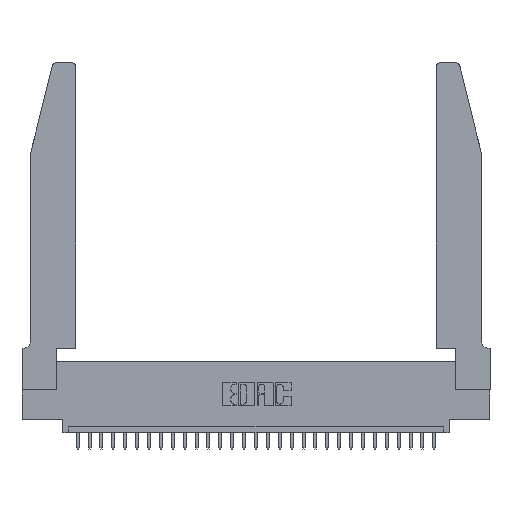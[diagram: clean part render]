
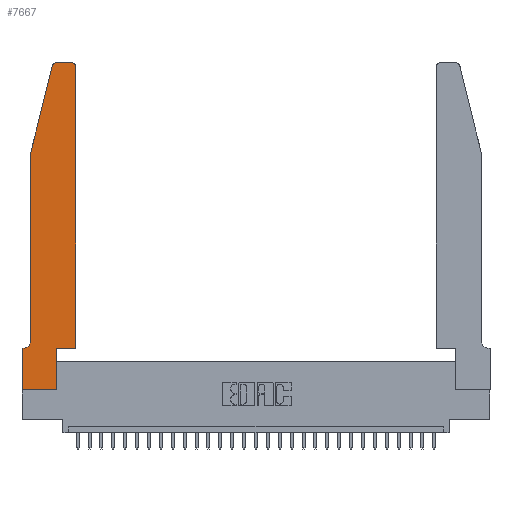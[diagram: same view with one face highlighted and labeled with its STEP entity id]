
A CAD part, top view. The second image highlights one B-rep face of the part: STEP entity #7667.
In plain terms, the highlighted planar face has unit normal (0, 0, 1).
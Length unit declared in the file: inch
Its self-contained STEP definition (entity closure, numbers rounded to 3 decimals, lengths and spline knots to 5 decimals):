
#286 = CARTESIAN_POINT ( 'NONE',  ( 0.2865, 0.35, 0.37 ) ) ;
#939 = VERTEX_POINT ( 'NONE', #19183 ) ;
#998 = ORIENTED_EDGE ( 'NONE', *, *, #2613, .T. ) ;
#1037 = DIRECTION ( 'NONE',  ( 0., -1., 0. ) ) ;
#2097 = DIRECTION ( 'NONE',  ( -1., 0., 0. ) ) ;
#2225 = DIRECTION ( 'NONE',  ( -1., 0., 0. ) ) ;
#2613 = EDGE_CURVE ( 'NONE', #14216, #12177, #20416, .T. ) ;
#2931 = CARTESIAN_POINT ( 'NONE',  ( 0.4205, 2.72, 0.37 ) ) ;
#3018 = CIRCLE ( 'NONE', #9901, 0.03 ) ;
#3137 = DIRECTION ( 'NONE',  ( 0., 1., 0. ) ) ;
#3200 = VECTOR ( 'NONE', #1037, 39.37008 ) ;
#3619 = DIRECTION ( 'NONE',  ( 0., 0., -1. ) ) ;
#3767 = DIRECTION ( 'NONE',  ( 1., 0., 0. ) ) ;
#3789 = EDGE_LOOP ( 'NONE', ( #17367, #20407, #10611, #998, #13333, #12583, #29360, #24971, #9728, #26779, #10005, #27233 ) ) ;
#3909 = CARTESIAN_POINT ( 'NONE',  ( 0.2865, 0., 0.37 ) ) ;
#3912 = CARTESIAN_POINT ( 'NONE',  ( 0.0755, 2., 0.37 ) ) ;
#4201 = CARTESIAN_POINT ( 'NONE',  ( 0., 0., 0.37 ) ) ;
#4343 = CARTESIAN_POINT ( 'NONE',  ( 0.4505, 0.35, 0.37 ) ) ;
#4499 = LINE ( 'NONE', #4343, #17440 ) ;
#5160 = VECTOR ( 'NONE', #19222, 39.37008 ) ;
#5215 = DIRECTION ( 'NONE',  ( 1., 0., 0. ) ) ;
#5331 = EDGE_CURVE ( 'NONE', #27801, #14195, #3018, .T. ) ;
#5688 = LINE ( 'NONE', #21274, #18525 ) ;
#6312 = CARTESIAN_POINT ( 'NONE',  ( 0.4505, 0.35, 0.37 ) ) ;
#6577 = VERTEX_POINT ( 'NONE', #15062 ) ;
#7338 = CARTESIAN_POINT ( 'NONE',  ( 0.284, 2.75, 0.37 ) ) ;
#7594 = DIRECTION ( 'NONE',  ( 1., 0., 0. ) ) ;
#7667 = ADVANCED_FACE ( 'NONE', ( #29215 ), #26389, .T. ) ;
#8290 = EDGE_CURVE ( 'NONE', #15858, #14216, #28092, .T. ) ;
#8324 = EDGE_CURVE ( 'NONE', #6577, #10058, #9838, .T. ) ;
#8410 = DIRECTION ( 'NONE',  ( 0., 0., 1. ) ) ;
#9519 = CARTESIAN_POINT ( 'NONE',  ( 0.0755, 0.35, 0.37 ) ) ;
#9728 = ORIENTED_EDGE ( 'NONE', *, *, #12633, .T. ) ;
#9838 = LINE ( 'NONE', #9519, #14478 ) ;
#9901 = AXIS2_PLACEMENT_3D ( 'NONE', #2931, #14165, #7594 ) ;
#10005 = ORIENTED_EDGE ( 'NONE', *, *, #25368, .T. ) ;
#10027 = CARTESIAN_POINT ( 'NONE',  ( 0.284, 2.72, 0.37 ) ) ;
#10058 = VERTEX_POINT ( 'NONE', #18893 ) ;
#10611 = ORIENTED_EDGE ( 'NONE', *, *, #8290, .T. ) ;
#10783 = CARTESIAN_POINT ( 'NONE',  ( 0.4505, 2.72, 0.37 ) ) ;
#11080 = EDGE_CURVE ( 'NONE', #10058, #28097, #27250, .T. ) ;
#12177 = VERTEX_POINT ( 'NONE', #17388 ) ;
#12583 = ORIENTED_EDGE ( 'NONE', *, *, #8324, .T. ) ;
#12633 = EDGE_CURVE ( 'NONE', #23079, #20661, #5688, .T. ) ;
#13333 = ORIENTED_EDGE ( 'NONE', *, *, #16205, .T. ) ;
#14165 = DIRECTION ( 'NONE',  ( 0., 0., 1. ) ) ;
#14195 = VERTEX_POINT ( 'NONE', #18794 ) ;
#14216 = VERTEX_POINT ( 'NONE', #28808 ) ;
#14478 = VECTOR ( 'NONE', #2225, 39.37008 ) ;
#14730 = AXIS2_PLACEMENT_3D ( 'NONE', #28827, #8410, #3767 ) ;
#15062 = CARTESIAN_POINT ( 'NONE',  ( 0.0055, 0.35, 0.37 ) ) ;
#15206 = VECTOR ( 'NONE', #29356, 39.37008 ) ;
#15331 = EDGE_CURVE ( 'NONE', #28097, #23079, #24478, .T. ) ;
#15646 = VECTOR ( 'NONE', #24870, 39.37008 ) ;
#15858 = VERTEX_POINT ( 'NONE', #28905 ) ;
#16205 = EDGE_CURVE ( 'NONE', #12177, #6577, #18338, .T. ) ;
#17106 = LINE ( 'NONE', #20157, #22124 ) ;
#17367 = ORIENTED_EDGE ( 'NONE', *, *, #24554, .T. ) ;
#17388 = CARTESIAN_POINT ( 'NONE',  ( 0.0755, 0.42, 0.37 ) ) ;
#17440 = VECTOR ( 'NONE', #23041, 39.37008 ) ;
#17623 = EDGE_CURVE ( 'NONE', #20661, #939, #4499, .T. ) ;
#18338 = CIRCLE ( 'NONE', #27350, 0.07 ) ;
#18358 = CARTESIAN_POINT ( 'NONE',  ( 0.0055, 0.42, 0.37 ) ) ;
#18525 = VECTOR ( 'NONE', #3137, 39.37008 ) ;
#18794 = CARTESIAN_POINT ( 'NONE',  ( 0.4205, 2.75, 0.37 ) ) ;
#18893 = CARTESIAN_POINT ( 'NONE',  ( 0., 0.35, 0.37 ) ) ;
#18998 = VECTOR ( 'NONE', #20796, 39.37008 ) ;
#19153 = VERTEX_POINT ( 'NONE', #7338 ) ;
#19183 = CARTESIAN_POINT ( 'NONE',  ( 0.4505, 0.35, 0.37 ) ) ;
#19222 = DIRECTION ( 'NONE',  ( 1., 0., 0. ) ) ;
#19464 = CARTESIAN_POINT ( 'NONE',  ( 0.0755, 2., 0.37 ) ) ;
#20157 = CARTESIAN_POINT ( 'NONE',  ( 0.2605, 2.75, 0.37 ) ) ;
#20407 = ORIENTED_EDGE ( 'NONE', *, *, #26977, .T. ) ;
#20416 = LINE ( 'NONE', #19464, #3200 ) ;
#20661 = VERTEX_POINT ( 'NONE', #286 ) ;
#20796 = DIRECTION ( 'NONE',  ( 0., -1., 0. ) ) ;
#21227 = CIRCLE ( 'NONE', #28475, 0.03 ) ;
#21274 = CARTESIAN_POINT ( 'NONE',  ( 0.2865, 0.35, 0.37 ) ) ;
#21605 = CARTESIAN_POINT ( 'NONE',  ( 0., 0., 0.37 ) ) ;
#22124 = VECTOR ( 'NONE', #22923, 39.37008 ) ;
#22923 = DIRECTION ( 'NONE',  ( -1., 0., 0. ) ) ;
#23041 = DIRECTION ( 'NONE',  ( 1., 0., 0. ) ) ;
#23079 = VERTEX_POINT ( 'NONE', #3909 ) ;
#23511 = DIRECTION ( 'NONE',  ( 0., 0., 1. ) ) ;
#24097 = CARTESIAN_POINT ( 'NONE',  ( 0., 0., 0.37 ) ) ;
#24478 = LINE ( 'NONE', #24097, #5160 ) ;
#24554 = EDGE_CURVE ( 'NONE', #14195, #19153, #17106, .T. ) ;
#24870 = DIRECTION ( 'NONE',  ( 0., 1., 0. ) ) ;
#24971 = ORIENTED_EDGE ( 'NONE', *, *, #15331, .T. ) ;
#25368 = EDGE_CURVE ( 'NONE', #939, #27801, #28548, .T. ) ;
#26389 = PLANE ( 'NONE',  #14730 ) ;
#26779 = ORIENTED_EDGE ( 'NONE', *, *, #17623, .T. ) ;
#26977 = EDGE_CURVE ( 'NONE', #19153, #15858, #21227, .T. ) ;
#27233 = ORIENTED_EDGE ( 'NONE', *, *, #5331, .T. ) ;
#27250 = LINE ( 'NONE', #21605, #18998 ) ;
#27350 = AXIS2_PLACEMENT_3D ( 'NONE', #18358, #3619, #2097 ) ;
#27801 = VERTEX_POINT ( 'NONE', #10783 ) ;
#28092 = LINE ( 'NONE', #3912, #15206 ) ;
#28097 = VERTEX_POINT ( 'NONE', #4201 ) ;
#28475 = AXIS2_PLACEMENT_3D ( 'NONE', #10027, #23511, #5215 ) ;
#28548 = LINE ( 'NONE', #6312, #15646 ) ;
#28808 = CARTESIAN_POINT ( 'NONE',  ( 0.0755, 2., 0.37 ) ) ;
#28827 = CARTESIAN_POINT ( 'NONE',  ( 0., 0.35, 0.37 ) ) ;
#28905 = CARTESIAN_POINT ( 'NONE',  ( 0.25487, 2.72718, 0.37 ) ) ;
#29215 = FACE_OUTER_BOUND ( 'NONE', #3789, .T. ) ;
#29356 = DIRECTION ( 'NONE',  ( -0.239, -0.971, 0. ) ) ;
#29360 = ORIENTED_EDGE ( 'NONE', *, *, #11080, .T. ) ;
